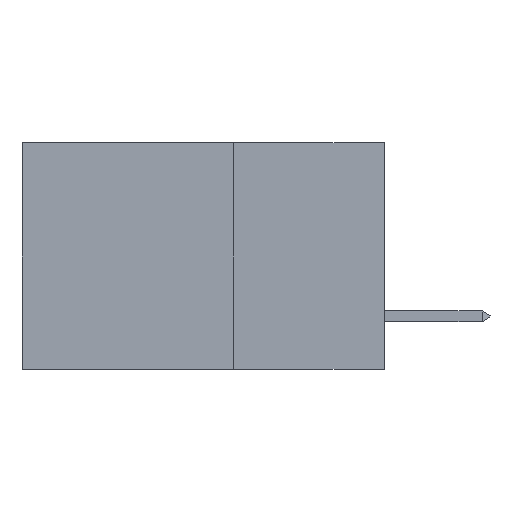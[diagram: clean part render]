
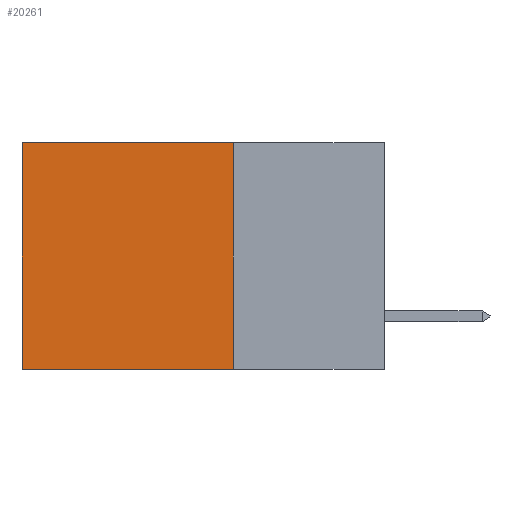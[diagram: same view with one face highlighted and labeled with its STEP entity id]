
A CAD part, left-side view. The second image highlights one B-rep face of the part: STEP entity #20261.
In plain terms, the highlighted planar face has unit normal (-1, 0, 0).
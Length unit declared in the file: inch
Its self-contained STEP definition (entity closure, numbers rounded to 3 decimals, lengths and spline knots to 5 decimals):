
#204 = CARTESIAN_POINT ( 'NONE',  ( 0.2875, 0.25, 0. ) ) ;
#473 = VERTEX_POINT ( 'NONE', #6541 ) ;
#1157 = DIRECTION ( 'NONE',  ( 0., 0., -1. ) ) ;
#1563 = CARTESIAN_POINT ( 'NONE',  ( 0.2875, 0.25, -0.375 ) ) ;
#1653 = VERTEX_POINT ( 'NONE', #204 ) ;
#2172 = EDGE_CURVE ( 'NONE', #14415, #473, #18403, .T. ) ;
#2885 = DIRECTION ( 'NONE',  ( 0., 1., 0. ) ) ;
#2905 = DIRECTION ( 'NONE',  ( 1., 0., 0. ) ) ;
#2973 = PLANE ( 'NONE',  #20081 ) ;
#3035 = FACE_OUTER_BOUND ( 'NONE', #12280, .T. ) ;
#4157 = CARTESIAN_POINT ( 'NONE',  ( 0.2875, 0.25, 0. ) ) ;
#4448 = CARTESIAN_POINT ( 'NONE',  ( 0.2875, 0.25, -0.375 ) ) ;
#4578 = EDGE_CURVE ( 'NONE', #1653, #10374, #7886, .T. ) ;
#4706 = VECTOR ( 'NONE', #7930, 39.37008 ) ;
#5856 = ORIENTED_EDGE ( 'NONE', *, *, #2172, .T. ) ;
#6541 = CARTESIAN_POINT ( 'NONE',  ( 0.2875, 0.6, -0.375 ) ) ;
#7149 = VECTOR ( 'NONE', #15497, 39.37008 ) ;
#7375 = VECTOR ( 'NONE', #7492, 39.37008 ) ;
#7492 = DIRECTION ( 'NONE',  ( 0., 0., -1. ) ) ;
#7652 = VECTOR ( 'NONE', #2885, 39.37008 ) ;
#7886 = LINE ( 'NONE', #4448, #7375 ) ;
#7930 = DIRECTION ( 'NONE',  ( 0., 0., -1. ) ) ;
#8625 = ORIENTED_EDGE ( 'NONE', *, *, #15908, .F. ) ;
#9171 = LINE ( 'NONE', #15918, #7652 ) ;
#10374 = VERTEX_POINT ( 'NONE', #1563 ) ;
#12134 = CARTESIAN_POINT ( 'NONE',  ( 0.2875, 0.6, 0. ) ) ;
#12280 = EDGE_LOOP ( 'NONE', ( #5856, #8625, #14690, #18813 ) ) ;
#14415 = VERTEX_POINT ( 'NONE', #12134 ) ;
#14690 = ORIENTED_EDGE ( 'NONE', *, *, #4578, .F. ) ;
#15497 = DIRECTION ( 'NONE',  ( 0., 1., 0. ) ) ;
#15815 = EDGE_CURVE ( 'NONE', #1653, #14415, #18567, .T. ) ;
#15908 = EDGE_CURVE ( 'NONE', #10374, #473, #9171, .T. ) ;
#15918 = CARTESIAN_POINT ( 'NONE',  ( 0.2875, 0.25, -0.375 ) ) ;
#16095 = CARTESIAN_POINT ( 'NONE',  ( 0.2875, 0.6, -0.375 ) ) ;
#18403 = LINE ( 'NONE', #16095, #4706 ) ;
#18567 = LINE ( 'NONE', #4157, #7149 ) ;
#18813 = ORIENTED_EDGE ( 'NONE', *, *, #15815, .T. ) ;
#18984 = CARTESIAN_POINT ( 'NONE',  ( 0.2875, 0.25, -0.375 ) ) ;
#20081 = AXIS2_PLACEMENT_3D ( 'NONE', #18984, #2905, #1157 ) ;
#20261 = ADVANCED_FACE ( 'NONE', ( #3035 ), #2973, .F. ) ;
